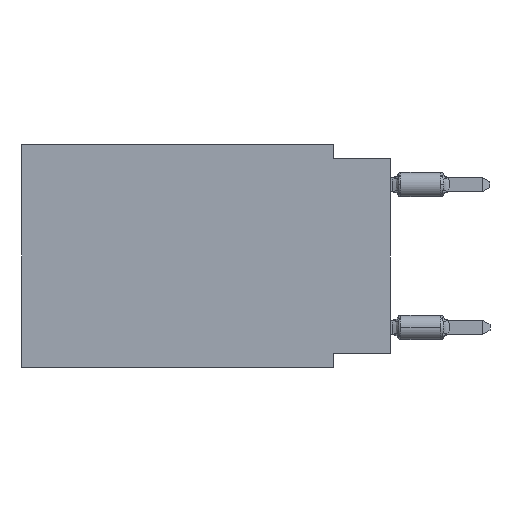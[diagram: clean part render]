
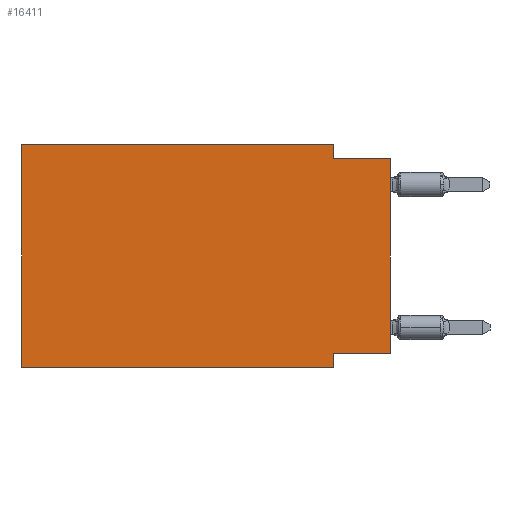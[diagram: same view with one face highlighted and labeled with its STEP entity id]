
A CAD part, left-side view. The second image highlights one B-rep face of the part: STEP entity #16411.
In plain terms, the highlighted planar face has unit normal (-1, 0, 0).
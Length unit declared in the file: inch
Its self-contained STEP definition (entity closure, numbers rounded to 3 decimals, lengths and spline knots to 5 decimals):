
#381 = VERTEX_POINT ( 'NONE', #1988 ) ;
#577 = LINE ( 'NONE', #7239, #2877 ) ;
#1397 = EDGE_CURVE ( 'NONE', #6777, #7327, #577, .T. ) ;
#1457 = VECTOR ( 'NONE', #7557, 39.37008 ) ;
#1970 = VECTOR ( 'NONE', #5236, 39.37008 ) ;
#1988 = CARTESIAN_POINT ( 'NONE',  ( 0., 0.1, -0.025 ) ) ;
#2079 = EDGE_CURVE ( 'NONE', #6777, #8200, #8074, .T. ) ;
#2222 = ORIENTED_EDGE ( 'NONE', *, *, #17141, .F. ) ;
#2672 = ORIENTED_EDGE ( 'NONE', *, *, #1397, .T. ) ;
#2877 = VECTOR ( 'NONE', #16580, 39.37008 ) ;
#3193 = CARTESIAN_POINT ( 'NONE',  ( 0., 0., -0.365 ) ) ;
#3852 = CARTESIAN_POINT ( 'NONE',  ( 0., 0.1, -0.39 ) ) ;
#4006 = CARTESIAN_POINT ( 'NONE',  ( 0., 0., -0.025 ) ) ;
#4175 = CARTESIAN_POINT ( 'NONE',  ( 0., 0.645, 0. ) ) ;
#4660 = VERTEX_POINT ( 'NONE', #16461 ) ;
#5236 = DIRECTION ( 'NONE',  ( 0., -1., 0. ) ) ;
#5377 = ORIENTED_EDGE ( 'NONE', *, *, #2079, .F. ) ;
#5442 = VECTOR ( 'NONE', #11248, 39.37008 ) ;
#5799 = ORIENTED_EDGE ( 'NONE', *, *, #6888, .F. ) ;
#5841 = EDGE_CURVE ( 'NONE', #4660, #381, #13821, .T. ) ;
#5993 = CARTESIAN_POINT ( 'NONE',  ( 0., 0.645, -0.39 ) ) ;
#6712 = VECTOR ( 'NONE', #16504, 39.37008 ) ;
#6777 = VERTEX_POINT ( 'NONE', #3193 ) ;
#6888 = EDGE_CURVE ( 'NONE', #14390, #15262, #9231, .T. ) ;
#7175 = LINE ( 'NONE', #12572, #5442 ) ;
#7213 = VECTOR ( 'NONE', #15309, 39.37008 ) ;
#7239 = CARTESIAN_POINT ( 'NONE',  ( 0., 0., 0. ) ) ;
#7327 = VERTEX_POINT ( 'NONE', #15663 ) ;
#7557 = DIRECTION ( 'NONE',  ( 0., 0., 1. ) ) ;
#7810 = CARTESIAN_POINT ( 'NONE',  ( 0., 0.645, 0. ) ) ;
#7828 = AXIS2_PLACEMENT_3D ( 'NONE', #10352, #12830, #15746 ) ;
#8074 = LINE ( 'NONE', #15946, #11874 ) ;
#8090 = ORIENTED_EDGE ( 'NONE', *, *, #5841, .F. ) ;
#8200 = VERTEX_POINT ( 'NONE', #14365 ) ;
#8481 = LINE ( 'NONE', #9809, #6712 ) ;
#8841 = EDGE_CURVE ( 'NONE', #8200, #16091, #7175, .T. ) ;
#9231 = LINE ( 'NONE', #7810, #1457 ) ;
#9809 = CARTESIAN_POINT ( 'NONE',  ( 0., 0.645, -0.39 ) ) ;
#9840 = CARTESIAN_POINT ( 'NONE',  ( 0., 0.1, 0. ) ) ;
#10352 = CARTESIAN_POINT ( 'NONE',  ( 0., 0.645, 0. ) ) ;
#11248 = DIRECTION ( 'NONE',  ( 0., 0., -1. ) ) ;
#11288 = ORIENTED_EDGE ( 'NONE', *, *, #8841, .F. ) ;
#11874 = VECTOR ( 'NONE', #14706, 39.37008 ) ;
#11888 = EDGE_CURVE ( 'NONE', #381, #7327, #13542, .T. ) ;
#12134 = DIRECTION ( 'NONE',  ( 0., -1., 0. ) ) ;
#12170 = ORIENTED_EDGE ( 'NONE', *, *, #11888, .F. ) ;
#12572 = CARTESIAN_POINT ( 'NONE',  ( 0., 0.1, -0.39 ) ) ;
#12830 = DIRECTION ( 'NONE',  ( 1., 0., 0. ) ) ;
#13542 = LINE ( 'NONE', #4006, #17331 ) ;
#13821 = LINE ( 'NONE', #9840, #7213 ) ;
#13835 = ORIENTED_EDGE ( 'NONE', *, *, #16492, .T. ) ;
#14365 = CARTESIAN_POINT ( 'NONE',  ( 0., 0.1, -0.365 ) ) ;
#14390 = VERTEX_POINT ( 'NONE', #5993 ) ;
#14675 = CARTESIAN_POINT ( 'NONE',  ( 0., 0.645, 0. ) ) ;
#14706 = DIRECTION ( 'NONE',  ( 0., 1., 0. ) ) ;
#14762 = LINE ( 'NONE', #4175, #1970 ) ;
#15262 = VERTEX_POINT ( 'NONE', #14675 ) ;
#15309 = DIRECTION ( 'NONE',  ( 0., 0., -1. ) ) ;
#15480 = PLANE ( 'NONE',  #7828 ) ;
#15596 = EDGE_LOOP ( 'NONE', ( #2672, #12170, #8090, #2222, #5799, #13835, #11288, #5377 ) ) ;
#15663 = CARTESIAN_POINT ( 'NONE',  ( 0., 0., -0.025 ) ) ;
#15746 = DIRECTION ( 'NONE',  ( 0., 0., -1. ) ) ;
#15946 = CARTESIAN_POINT ( 'NONE',  ( 0., 0., -0.365 ) ) ;
#16091 = VERTEX_POINT ( 'NONE', #3852 ) ;
#16411 = ADVANCED_FACE ( 'NONE', ( #16873 ), #15480, .F. ) ;
#16461 = CARTESIAN_POINT ( 'NONE',  ( 0., 0.1, 0. ) ) ;
#16492 = EDGE_CURVE ( 'NONE', #14390, #16091, #8481, .T. ) ;
#16504 = DIRECTION ( 'NONE',  ( 0., -1., 0. ) ) ;
#16580 = DIRECTION ( 'NONE',  ( 0., 0., 1. ) ) ;
#16873 = FACE_OUTER_BOUND ( 'NONE', #15596, .T. ) ;
#17141 = EDGE_CURVE ( 'NONE', #15262, #4660, #14762, .T. ) ;
#17331 = VECTOR ( 'NONE', #12134, 39.37008 ) ;
